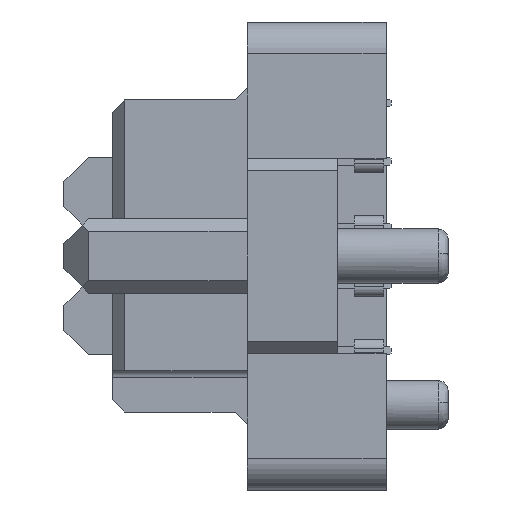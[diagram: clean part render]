
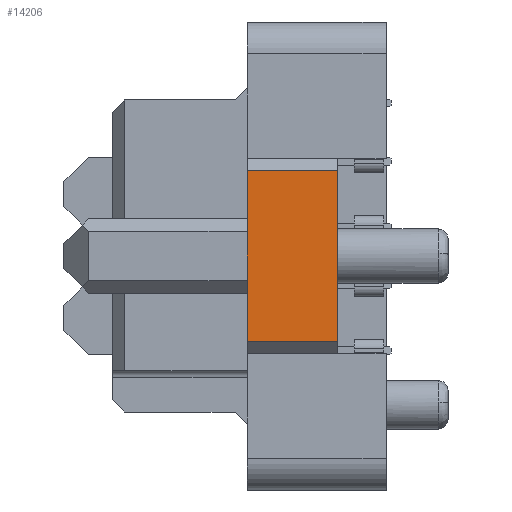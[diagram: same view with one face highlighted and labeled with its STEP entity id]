
A CAD part, left-side view. The second image highlights one B-rep face of the part: STEP entity #14206.
In plain terms, the highlighted planar face has unit normal (-1, 0, 0).
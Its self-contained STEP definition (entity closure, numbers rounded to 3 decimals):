
#452 = CARTESIAN_POINT ( 'NONE',  ( -16.09, -0.925, 0. ) ) ;
#516 = ORIENTED_EDGE ( 'NONE', *, *, #6207, .F. ) ;
#1402 = CARTESIAN_POINT ( 'NONE',  ( -16.09, -0.925, -1.75 ) ) ;
#2526 = VERTEX_POINT ( 'NONE', #76134 ) ;
#2855 = DIRECTION ( 'NONE',  ( 0., 1., 0. ) ) ;
#3534 = VECTOR ( 'NONE', #56497, 1000. ) ;
#6207 = EDGE_CURVE ( 'NONE', #58598, #66281, #62192, .T. ) ;
#7347 = DIRECTION ( 'NONE',  ( 1., 0., 0. ) ) ;
#7811 = PLANE ( 'NONE',  #79254 ) ;
#14206 = ADVANCED_FACE ( 'NONE', ( #75461 ), #7811, .F. ) ;
#18762 = CARTESIAN_POINT ( 'NONE',  ( -16.09, -1.85, 0. ) ) ;
#21708 = LINE ( 'NONE', #95752, #95777 ) ;
#22468 = EDGE_CURVE ( 'NONE', #58598, #38398, #47719, .T. ) ;
#23988 = DIRECTION ( 'NONE',  ( 0., 1., 0. ) ) ;
#26277 = ORIENTED_EDGE ( 'NONE', *, *, #22468, .T. ) ;
#38398 = VERTEX_POINT ( 'NONE', #89526 ) ;
#47181 = EDGE_CURVE ( 'NONE', #66281, #2526, #82228, .T. ) ;
#47719 = LINE ( 'NONE', #18762, #3534 ) ;
#50318 = VECTOR ( 'NONE', #63044, 1000. ) ;
#51136 = DIRECTION ( 'NONE',  ( 0., -1., 0. ) ) ;
#55390 = CARTESIAN_POINT ( 'NONE',  ( -16.09, 0., -1.75 ) ) ;
#56497 = DIRECTION ( 'NONE',  ( 0., 0., 1. ) ) ;
#58598 = VERTEX_POINT ( 'NONE', #68214 ) ;
#62192 = LINE ( 'NONE', #1402, #81302 ) ;
#63044 = DIRECTION ( 'NONE',  ( 0., 0., 1. ) ) ;
#66281 = VERTEX_POINT ( 'NONE', #55390 ) ;
#68214 = CARTESIAN_POINT ( 'NONE',  ( -16.09, -1.85, -1.75 ) ) ;
#75461 = FACE_OUTER_BOUND ( 'NONE', #87343, .T. ) ;
#76134 = CARTESIAN_POINT ( 'NONE',  ( -16.09, 0., 1.75 ) ) ;
#79254 = AXIS2_PLACEMENT_3D ( 'NONE', #452, #7347, #23988 ) ;
#79283 = ORIENTED_EDGE ( 'NONE', *, *, #47181, .F. ) ;
#81302 = VECTOR ( 'NONE', #2855, 1000. ) ;
#82071 = EDGE_CURVE ( 'NONE', #2526, #38398, #21708, .T. ) ;
#82228 = LINE ( 'NONE', #92972, #50318 ) ;
#87343 = EDGE_LOOP ( 'NONE', ( #88821, #79283, #516, #26277 ) ) ;
#88821 = ORIENTED_EDGE ( 'NONE', *, *, #82071, .F. ) ;
#89526 = CARTESIAN_POINT ( 'NONE',  ( -16.09, -1.85, 1.75 ) ) ;
#92972 = CARTESIAN_POINT ( 'NONE',  ( -16.09, 0., 0. ) ) ;
#95752 = CARTESIAN_POINT ( 'NONE',  ( -16.09, -0.925, 1.75 ) ) ;
#95777 = VECTOR ( 'NONE', #51136, 1000. ) ;
